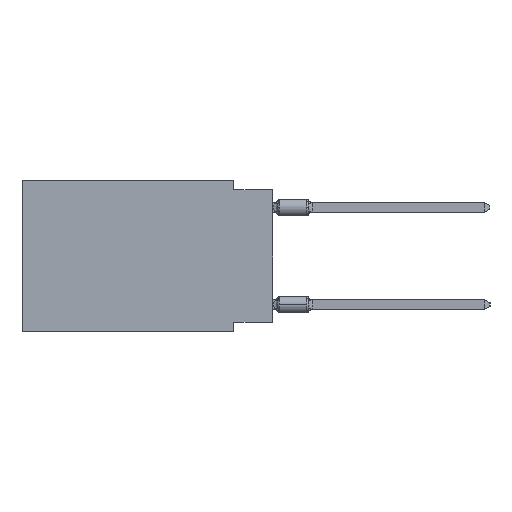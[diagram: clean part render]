
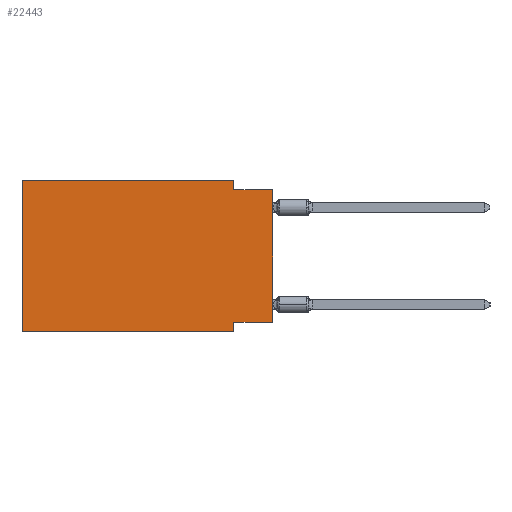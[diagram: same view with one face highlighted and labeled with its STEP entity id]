
A CAD part, left-side view. The second image highlights one B-rep face of the part: STEP entity #22443.
In plain terms, the highlighted planar face has unit normal (-1, 0, 0).
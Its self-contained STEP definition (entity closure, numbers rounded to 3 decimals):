
#350 = EDGE_LOOP ( 'NONE', ( #31335, #15516, #19159, #16559, #17597, #11327, #25310, #31382 ) ) ;
#559 = CARTESIAN_POINT ( 'NONE',  ( 0., 0., -0.635 ) ) ;
#831 = CARTESIAN_POINT ( 'NONE',  ( 0., 0., -0.635 ) ) ;
#1728 = CARTESIAN_POINT ( 'NONE',  ( 0., 16.383, 0. ) ) ;
#1758 = DIRECTION ( 'NONE',  ( 0., 0., 1. ) ) ;
#1901 = PLANE ( 'NONE',  #34758 ) ;
#3393 = EDGE_CURVE ( 'NONE', #15046, #13013, #35487, .T. ) ;
#4250 = LINE ( 'NONE', #15431, #24626 ) ;
#4339 = DIRECTION ( 'NONE',  ( 0., 0., -1. ) ) ;
#4542 = DIRECTION ( 'NONE',  ( 0., -1., 0. ) ) ;
#5273 = CARTESIAN_POINT ( 'NONE',  ( 0., 2.54, -0.635 ) ) ;
#5313 = CARTESIAN_POINT ( 'NONE',  ( 0., 2.54, -9.906 ) ) ;
#6275 = EDGE_CURVE ( 'NONE', #22878, #25868, #30818, .T. ) ;
#7616 = EDGE_CURVE ( 'NONE', #12091, #15046, #19937, .T. ) ;
#9989 = DIRECTION ( 'NONE',  ( 0., -1., 0. ) ) ;
#11327 = ORIENTED_EDGE ( 'NONE', *, *, #22452, .T. ) ;
#11339 = EDGE_CURVE ( 'NONE', #14191, #32493, #12552, .T. ) ;
#11756 = DIRECTION ( 'NONE',  ( 0., 0., 1. ) ) ;
#12091 = VERTEX_POINT ( 'NONE', #27819 ) ;
#12552 = LINE ( 'NONE', #26548, #35750 ) ;
#13013 = VERTEX_POINT ( 'NONE', #16992 ) ;
#14191 = VERTEX_POINT ( 'NONE', #26246 ) ;
#14353 = EDGE_CURVE ( 'NONE', #14191, #22878, #4250, .T. ) ;
#15046 = VERTEX_POINT ( 'NONE', #31005 ) ;
#15296 = VECTOR ( 'NONE', #11756, 1000. ) ;
#15431 = CARTESIAN_POINT ( 'NONE',  ( 0., 0., -9.271 ) ) ;
#15516 = ORIENTED_EDGE ( 'NONE', *, *, #21258, .F. ) ;
#16150 = CARTESIAN_POINT ( 'NONE',  ( 0., 2.54, -9.271 ) ) ;
#16241 = VECTOR ( 'NONE', #4542, 1000. ) ;
#16559 = ORIENTED_EDGE ( 'NONE', *, *, #3393, .F. ) ;
#16649 = DIRECTION ( 'NONE',  ( 0., 0., -1. ) ) ;
#16992 = CARTESIAN_POINT ( 'NONE',  ( 0., 2.54, 0. ) ) ;
#17597 = ORIENTED_EDGE ( 'NONE', *, *, #7616, .F. ) ;
#18360 = CARTESIAN_POINT ( 'NONE',  ( 0., 16.383, 0. ) ) ;
#18856 = DIRECTION ( 'NONE',  ( 0., -1., 0. ) ) ;
#19159 = ORIENTED_EDGE ( 'NONE', *, *, #30663, .F. ) ;
#19184 = LINE ( 'NONE', #19379, #29540 ) ;
#19379 = CARTESIAN_POINT ( 'NONE',  ( 0., 2.54, 0. ) ) ;
#19937 = LINE ( 'NONE', #26272, #15296 ) ;
#20494 = CARTESIAN_POINT ( 'NONE',  ( 0., 2.54, -9.906 ) ) ;
#20659 = DIRECTION ( 'NONE',  ( 0., 1., 0. ) ) ;
#21258 = EDGE_CURVE ( 'NONE', #22580, #32493, #28772, .T. ) ;
#21453 = FACE_OUTER_BOUND ( 'NONE', #350, .T. ) ;
#21992 = DIRECTION ( 'NONE',  ( 0., 0., -1. ) ) ;
#22443 = ADVANCED_FACE ( 'NONE', ( #21453 ), #1901, .F. ) ;
#22452 = EDGE_CURVE ( 'NONE', #12091, #25868, #24437, .T. ) ;
#22580 = VERTEX_POINT ( 'NONE', #5273 ) ;
#22878 = VERTEX_POINT ( 'NONE', #16150 ) ;
#24437 = LINE ( 'NONE', #35784, #25247 ) ;
#24626 = VECTOR ( 'NONE', #20659, 1000. ) ;
#25247 = VECTOR ( 'NONE', #18856, 1000. ) ;
#25310 = ORIENTED_EDGE ( 'NONE', *, *, #6275, .F. ) ;
#25549 = VECTOR ( 'NONE', #9989, 1000. ) ;
#25868 = VERTEX_POINT ( 'NONE', #20494 ) ;
#26246 = CARTESIAN_POINT ( 'NONE',  ( 0., 0., -9.271 ) ) ;
#26272 = CARTESIAN_POINT ( 'NONE',  ( 0., 16.383, 0. ) ) ;
#26548 = CARTESIAN_POINT ( 'NONE',  ( 0., 0., 0. ) ) ;
#27728 = VECTOR ( 'NONE', #16649, 1000. ) ;
#27819 = CARTESIAN_POINT ( 'NONE',  ( 0., 16.383, -9.906 ) ) ;
#28772 = LINE ( 'NONE', #831, #16241 ) ;
#29540 = VECTOR ( 'NONE', #21992, 1000. ) ;
#29681 = DIRECTION ( 'NONE',  ( 1., 0., 0. ) ) ;
#30663 = EDGE_CURVE ( 'NONE', #13013, #22580, #19184, .T. ) ;
#30818 = LINE ( 'NONE', #5313, #27728 ) ;
#31005 = CARTESIAN_POINT ( 'NONE',  ( 0., 16.383, 0. ) ) ;
#31335 = ORIENTED_EDGE ( 'NONE', *, *, #11339, .T. ) ;
#31382 = ORIENTED_EDGE ( 'NONE', *, *, #14353, .F. ) ;
#32493 = VERTEX_POINT ( 'NONE', #559 ) ;
#34758 = AXIS2_PLACEMENT_3D ( 'NONE', #1728, #29681, #4339 ) ;
#35487 = LINE ( 'NONE', #18360, #25549 ) ;
#35750 = VECTOR ( 'NONE', #1758, 1000. ) ;
#35784 = CARTESIAN_POINT ( 'NONE',  ( 0., 16.383, -9.906 ) ) ;
